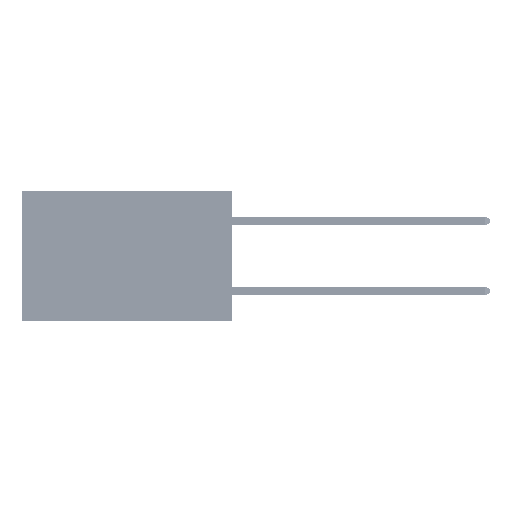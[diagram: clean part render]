
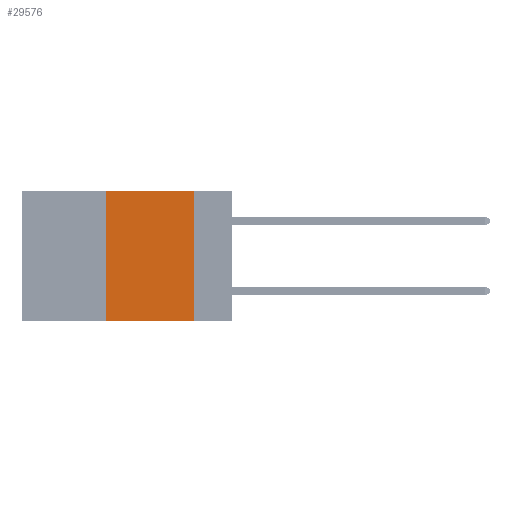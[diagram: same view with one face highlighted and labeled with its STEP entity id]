
A CAD part, left-side view. The second image highlights one B-rep face of the part: STEP entity #29576.
In plain terms, the highlighted planar face has unit normal (-1, 0, 0).
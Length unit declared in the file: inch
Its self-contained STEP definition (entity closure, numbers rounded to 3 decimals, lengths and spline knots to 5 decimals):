
#1798 = CARTESIAN_POINT ( 'NONE',  ( 0., 0.36, -0.37 ) ) ;
#2690 = VECTOR ( 'NONE', #9065, 39.37008 ) ;
#3518 = VERTEX_POINT ( 'NONE', #34016 ) ;
#3555 = EDGE_LOOP ( 'NONE', ( #51215, #44460, #34907, #40145 ) ) ;
#6459 = EDGE_CURVE ( 'NONE', #12014, #41526, #34013, .T. ) ;
#9065 = DIRECTION ( 'NONE',  ( 0., -1., 0. ) ) ;
#10245 = AXIS2_PLACEMENT_3D ( 'NONE', #32405, #20096, #22440 ) ;
#10438 = CARTESIAN_POINT ( 'NONE',  ( 0., 0.36, 0. ) ) ;
#11062 = CARTESIAN_POINT ( 'NONE',  ( 0., 0.11, -0.37 ) ) ;
#12014 = VERTEX_POINT ( 'NONE', #1798 ) ;
#13564 = DIRECTION ( 'NONE',  ( 0., 0., -1. ) ) ;
#16016 = CARTESIAN_POINT ( 'NONE',  ( 0., 0.36, 0. ) ) ;
#19723 = VECTOR ( 'NONE', #37700, 39.37008 ) ;
#20061 = EDGE_CURVE ( 'NONE', #41526, #3518, #45727, .T. ) ;
#20096 = DIRECTION ( 'NONE',  ( 1., 0., 0. ) ) ;
#21683 = VECTOR ( 'NONE', #13564, 39.37008 ) ;
#22440 = DIRECTION ( 'NONE',  ( 0., 0., -1. ) ) ;
#23821 = EDGE_CURVE ( 'NONE', #3518, #33132, #42135, .T. ) ;
#26124 = CARTESIAN_POINT ( 'NONE',  ( 0., 0.11, 0. ) ) ;
#27953 = PLANE ( 'NONE',  #10245 ) ;
#28465 = DIRECTION ( 'NONE',  ( 0., -1., 0. ) ) ;
#28816 = VECTOR ( 'NONE', #28465, 39.37008 ) ;
#29576 = ADVANCED_FACE ( 'NONE', ( #40289 ), #27953, .F. ) ;
#32146 = LINE ( 'NONE', #48138, #28816 ) ;
#32405 = CARTESIAN_POINT ( 'NONE',  ( 0., 0.6, 0. ) ) ;
#33132 = VERTEX_POINT ( 'NONE', #11062 ) ;
#33691 = EDGE_CURVE ( 'NONE', #12014, #33132, #32146, .T. ) ;
#34013 = LINE ( 'NONE', #10438, #19723 ) ;
#34016 = CARTESIAN_POINT ( 'NONE',  ( 0., 0.11, 0. ) ) ;
#34907 = ORIENTED_EDGE ( 'NONE', *, *, #6459, .F. ) ;
#37700 = DIRECTION ( 'NONE',  ( 0., 0., 1. ) ) ;
#37869 = CARTESIAN_POINT ( 'NONE',  ( 0., 0.6, 0. ) ) ;
#40145 = ORIENTED_EDGE ( 'NONE', *, *, #33691, .T. ) ;
#40289 = FACE_OUTER_BOUND ( 'NONE', #3555, .T. ) ;
#41526 = VERTEX_POINT ( 'NONE', #16016 ) ;
#42135 = LINE ( 'NONE', #26124, #21683 ) ;
#44460 = ORIENTED_EDGE ( 'NONE', *, *, #20061, .F. ) ;
#45727 = LINE ( 'NONE', #37869, #2690 ) ;
#48138 = CARTESIAN_POINT ( 'NONE',  ( 0., 0.6, -0.37 ) ) ;
#51215 = ORIENTED_EDGE ( 'NONE', *, *, #23821, .F. ) ;
